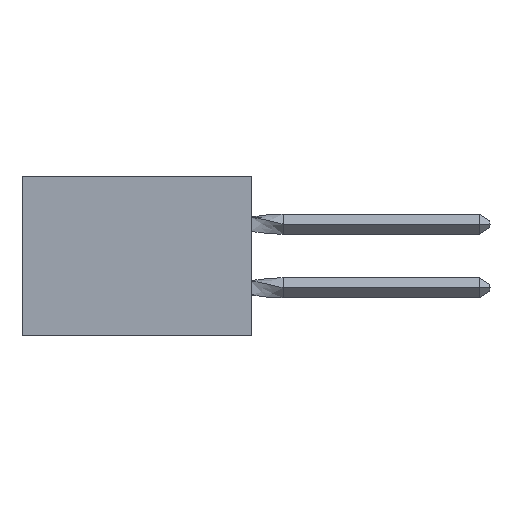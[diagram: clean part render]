
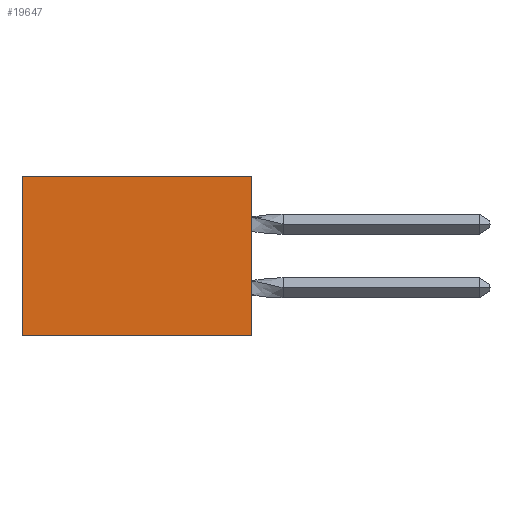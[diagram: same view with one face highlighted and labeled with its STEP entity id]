
A CAD part, left-side view. The second image highlights one B-rep face of the part: STEP entity #19647.
In plain terms, the highlighted planar face has unit normal (-1, 0, 0).
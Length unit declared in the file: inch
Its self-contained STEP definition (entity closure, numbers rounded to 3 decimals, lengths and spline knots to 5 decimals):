
#237 = CARTESIAN_POINT ( 'NONE',  ( 0.305, 0., 0. ) ) ;
#268 = ORIENTED_EDGE ( 'NONE', *, *, #4759, .T. ) ;
#323 = DIRECTION ( 'NONE',  ( 0., 1., 0. ) ) ;
#454 = ORIENTED_EDGE ( 'NONE', *, *, #18167, .F. ) ;
#1372 = DIRECTION ( 'NONE',  ( 0., 0., -1. ) ) ;
#3254 = VERTEX_POINT ( 'NONE', #22549 ) ;
#4718 = VECTOR ( 'NONE', #22261, 39.37008 ) ;
#4759 = EDGE_CURVE ( 'NONE', #24006, #3254, #12661, .T. ) ;
#5590 = VECTOR ( 'NONE', #1372, 39.37008 ) ;
#6348 = DIRECTION ( 'NONE',  ( 0., 0., -1. ) ) ;
#7149 = VECTOR ( 'NONE', #20831, 39.37008 ) ;
#7957 = CARTESIAN_POINT ( 'NONE',  ( 0.305, 0.72, -0.5 ) ) ;
#8979 = VERTEX_POINT ( 'NONE', #18012 ) ;
#9614 = VERTEX_POINT ( 'NONE', #22112 ) ;
#9957 = ORIENTED_EDGE ( 'NONE', *, *, #23087, .F. ) ;
#10550 = LINE ( 'NONE', #23346, #5590 ) ;
#11716 = ORIENTED_EDGE ( 'NONE', *, *, #12697, .T. ) ;
#11917 = CARTESIAN_POINT ( 'NONE',  ( 0.305, 0., -0.5 ) ) ;
#12661 = LINE ( 'NONE', #7957, #7149 ) ;
#12697 = EDGE_CURVE ( 'NONE', #9614, #24006, #23208, .T. ) ;
#13166 = CARTESIAN_POINT ( 'NONE',  ( 0.305, 0.72, 0. ) ) ;
#14287 = EDGE_LOOP ( 'NONE', ( #268, #9957, #454, #11716 ) ) ;
#15687 = VECTOR ( 'NONE', #323, 39.37008 ) ;
#18012 = CARTESIAN_POINT ( 'NONE',  ( 0.305, 0., -0.5 ) ) ;
#18167 = EDGE_CURVE ( 'NONE', #9614, #8979, #10550, .T. ) ;
#18232 = AXIS2_PLACEMENT_3D ( 'NONE', #11917, #19379, #6348 ) ;
#19379 = DIRECTION ( 'NONE',  ( 1., 0., 0. ) ) ;
#19647 = ADVANCED_FACE ( 'NONE', ( #22210 ), #20983, .F. ) ;
#20831 = DIRECTION ( 'NONE',  ( 0., 0., -1. ) ) ;
#20983 = PLANE ( 'NONE',  #18232 ) ;
#21236 = LINE ( 'NONE', #23831, #4718 ) ;
#22112 = CARTESIAN_POINT ( 'NONE',  ( 0.305, 0., 0. ) ) ;
#22210 = FACE_OUTER_BOUND ( 'NONE', #14287, .T. ) ;
#22261 = DIRECTION ( 'NONE',  ( 0., 1., 0. ) ) ;
#22549 = CARTESIAN_POINT ( 'NONE',  ( 0.305, 0.72, -0.5 ) ) ;
#23087 = EDGE_CURVE ( 'NONE', #8979, #3254, #21236, .T. ) ;
#23208 = LINE ( 'NONE', #237, #15687 ) ;
#23346 = CARTESIAN_POINT ( 'NONE',  ( 0.305, 0., -0.5 ) ) ;
#23831 = CARTESIAN_POINT ( 'NONE',  ( 0.305, 0., -0.5 ) ) ;
#24006 = VERTEX_POINT ( 'NONE', #13166 ) ;
